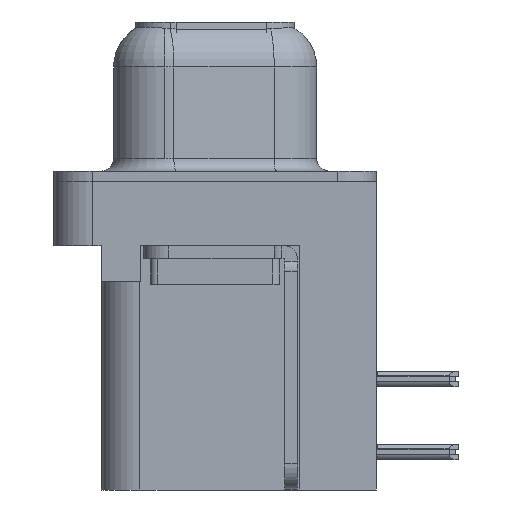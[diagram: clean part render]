
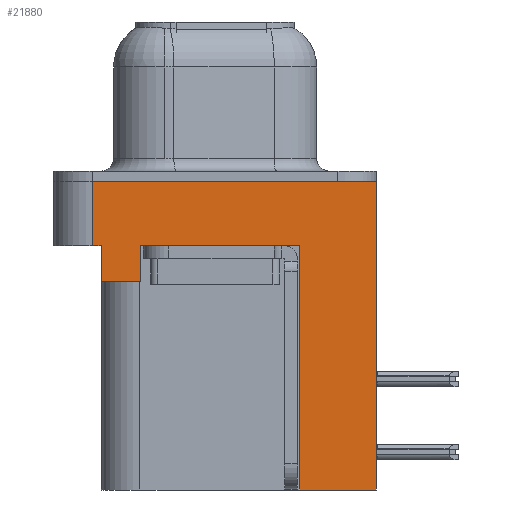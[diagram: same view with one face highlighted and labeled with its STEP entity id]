
A CAD part, left-side view. The second image highlights one B-rep face of the part: STEP entity #21880.
In plain terms, the highlighted planar face has unit normal (-1, 0, 0).
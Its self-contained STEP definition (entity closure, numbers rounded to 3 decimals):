
#513 = VECTOR ( 'NONE', #14817, 1000. ) ;
#533 = CARTESIAN_POINT ( 'NONE',  ( -3., -6.275, 0. ) ) ;
#1328 = ORIENTED_EDGE ( 'NONE', *, *, #2507, .F. ) ;
#1587 = LINE ( 'NONE', #16981, #15776 ) ;
#1885 = CARTESIAN_POINT ( 'NONE',  ( -3., -6.275, 0. ) ) ;
#2463 = CARTESIAN_POINT ( 'NONE',  ( -3., 4.425, -3.9 ) ) ;
#2507 = EDGE_CURVE ( 'NONE', #16142, #21212, #1587, .T. ) ;
#2525 = VERTEX_POINT ( 'NONE', #17086 ) ;
#2570 = DIRECTION ( 'NONE',  ( 0., 0., 1. ) ) ;
#3397 = EDGE_LOOP ( 'NONE', ( #25548, #1328, #23442, #5459, #28826, #6455, #30594, #19994, #3938, #17929 ) ) ;
#3938 = ORIENTED_EDGE ( 'NONE', *, *, #27869, .F. ) ;
#3965 = VERTEX_POINT ( 'NONE', #23389 ) ;
#4531 = PLANE ( 'NONE',  #29381 ) ;
#4986 = CARTESIAN_POINT ( 'NONE',  ( -3., -6.275, -2.5 ) ) ;
#5237 = EDGE_CURVE ( 'NONE', #16142, #17445, #8017, .T. ) ;
#5253 = VERTEX_POINT ( 'NONE', #12189 ) ;
#5266 = EDGE_CURVE ( 'NONE', #23886, #5253, #25977, .T. ) ;
#5459 = ORIENTED_EDGE ( 'NONE', *, *, #15340, .F. ) ;
#6075 = LINE ( 'NONE', #533, #20630 ) ;
#6337 = CARTESIAN_POINT ( 'NONE',  ( -3., -6.275, -2.5 ) ) ;
#6455 = ORIENTED_EDGE ( 'NONE', *, *, #7370, .T. ) ;
#7275 = DIRECTION ( 'NONE',  ( 0., 1., 0. ) ) ;
#7362 = DIRECTION ( 'NONE',  ( 0., 0., 1. ) ) ;
#7370 = EDGE_CURVE ( 'NONE', #26814, #23886, #28888, .T. ) ;
#8017 = LINE ( 'NONE', #6337, #24470 ) ;
#8219 = VERTEX_POINT ( 'NONE', #25085 ) ;
#8486 = EDGE_CURVE ( 'NONE', #8219, #9502, #15279, .T. ) ;
#9502 = VERTEX_POINT ( 'NONE', #1885 ) ;
#10752 = CARTESIAN_POINT ( 'NONE',  ( -3., 4.775, -2.5 ) ) ;
#11943 = CARTESIAN_POINT ( 'NONE',  ( -3., 4.425, -3.9 ) ) ;
#12000 = VECTOR ( 'NONE', #22849, 1000. ) ;
#12031 = CARTESIAN_POINT ( 'NONE',  ( -3., -6.275, -2.5 ) ) ;
#12189 = CARTESIAN_POINT ( 'NONE',  ( -3., -3.295, -2.5 ) ) ;
#12218 = CARTESIAN_POINT ( 'NONE',  ( -3., -3.295, -12. ) ) ;
#12327 = DIRECTION ( 'NONE',  ( 0., 0., 1. ) ) ;
#12583 = CARTESIAN_POINT ( 'NONE',  ( -3., 4.775, 0. ) ) ;
#13085 = CARTESIAN_POINT ( 'NONE',  ( -3., 4.425, -2.5 ) ) ;
#13364 = DIRECTION ( 'NONE',  ( 0., 0., 1. ) ) ;
#14817 = DIRECTION ( 'NONE',  ( 0., -1., 0. ) ) ;
#15279 = LINE ( 'NONE', #18085, #22027 ) ;
#15340 = EDGE_CURVE ( 'NONE', #2525, #17445, #28279, .T. ) ;
#15776 = VECTOR ( 'NONE', #29173, 1000. ) ;
#16142 = VERTEX_POINT ( 'NONE', #10752 ) ;
#16981 = CARTESIAN_POINT ( 'NONE',  ( -3., 4.775, -2.5 ) ) ;
#17086 = CARTESIAN_POINT ( 'NONE',  ( -3., 4.425, -3.9 ) ) ;
#17445 = VERTEX_POINT ( 'NONE', #13085 ) ;
#17929 = ORIENTED_EDGE ( 'NONE', *, *, #8486, .T. ) ;
#18085 = CARTESIAN_POINT ( 'NONE',  ( -3., -6.275, -2.5 ) ) ;
#19118 = DIRECTION ( 'NONE',  ( 0., -1., 0. ) ) ;
#19522 = LINE ( 'NONE', #12218, #20653 ) ;
#19809 = VECTOR ( 'NONE', #27546, 1000. ) ;
#19994 = ORIENTED_EDGE ( 'NONE', *, *, #26866, .F. ) ;
#20630 = VECTOR ( 'NONE', #22058, 1000. ) ;
#20653 = VECTOR ( 'NONE', #12327, 1000. ) ;
#21212 = VERTEX_POINT ( 'NONE', #12583 ) ;
#21831 = CARTESIAN_POINT ( 'NONE',  ( -3., 2.895, -2.5 ) ) ;
#21880 = ADVANCED_FACE ( 'NONE', ( #24136 ), #4531, .T. ) ;
#21928 = EDGE_CURVE ( 'NONE', #21212, #9502, #6075, .T. ) ;
#22027 = VECTOR ( 'NONE', #13364, 1000. ) ;
#22058 = DIRECTION ( 'NONE',  ( 0., -1., 0. ) ) ;
#22849 = DIRECTION ( 'NONE',  ( 0., 0., 1. ) ) ;
#23321 = CARTESIAN_POINT ( 'NONE',  ( -3., 2.895, -3.9 ) ) ;
#23389 = CARTESIAN_POINT ( 'NONE',  ( -3., -3.295, -12. ) ) ;
#23442 = ORIENTED_EDGE ( 'NONE', *, *, #5237, .T. ) ;
#23886 = VERTEX_POINT ( 'NONE', #21831 ) ;
#23941 = EDGE_CURVE ( 'NONE', #26814, #2525, #28980, .T. ) ;
#24098 = VECTOR ( 'NONE', #2570, 1000. ) ;
#24136 = FACE_OUTER_BOUND ( 'NONE', #3397, .T. ) ;
#24470 = VECTOR ( 'NONE', #19118, 1000. ) ;
#25040 = LINE ( 'NONE', #25100, #19809 ) ;
#25085 = CARTESIAN_POINT ( 'NONE',  ( -3., -6.275, -12. ) ) ;
#25100 = CARTESIAN_POINT ( 'NONE',  ( -3., -3.295, -12. ) ) ;
#25548 = ORIENTED_EDGE ( 'NONE', *, *, #21928, .F. ) ;
#25977 = LINE ( 'NONE', #4986, #513 ) ;
#26814 = VERTEX_POINT ( 'NONE', #23321 ) ;
#26866 = EDGE_CURVE ( 'NONE', #3965, #5253, #19522, .T. ) ;
#27546 = DIRECTION ( 'NONE',  ( 0., 1., 0. ) ) ;
#27869 = EDGE_CURVE ( 'NONE', #8219, #3965, #25040, .T. ) ;
#28279 = LINE ( 'NONE', #2463, #24098 ) ;
#28603 = VECTOR ( 'NONE', #7275, 1000. ) ;
#28826 = ORIENTED_EDGE ( 'NONE', *, *, #23941, .F. ) ;
#28888 = LINE ( 'NONE', #29845, #12000 ) ;
#28980 = LINE ( 'NONE', #11943, #28603 ) ;
#29173 = DIRECTION ( 'NONE',  ( 0., 0., 1. ) ) ;
#29381 = AXIS2_PLACEMENT_3D ( 'NONE', #12031, #30921, #7362 ) ;
#29845 = CARTESIAN_POINT ( 'NONE',  ( -3., 2.895, -3.9 ) ) ;
#30594 = ORIENTED_EDGE ( 'NONE', *, *, #5266, .T. ) ;
#30921 = DIRECTION ( 'NONE',  ( -1., 0., 0. ) ) ;
